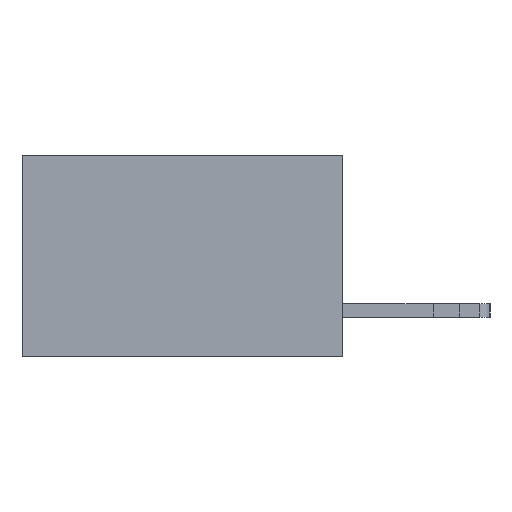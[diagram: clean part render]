
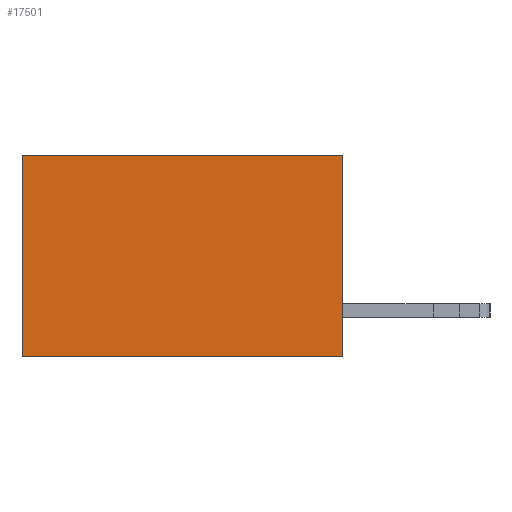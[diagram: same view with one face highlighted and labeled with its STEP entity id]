
A CAD part, left-side view. The second image highlights one B-rep face of the part: STEP entity #17501.
In plain terms, the highlighted planar face has unit normal (-1, 0, 0).
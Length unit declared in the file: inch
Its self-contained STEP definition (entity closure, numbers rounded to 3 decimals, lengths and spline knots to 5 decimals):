
#736 = VERTEX_POINT ( 'NONE', #9487 ) ;
#1729 = EDGE_CURVE ( 'NONE', #8625, #7861, #22455, .T. ) ;
#1842 = CARTESIAN_POINT ( 'NONE',  ( 0.277, 0., -0.37 ) ) ;
#3627 = CARTESIAN_POINT ( 'NONE',  ( 0.277, 0., -0.37 ) ) ;
#3672 = CARTESIAN_POINT ( 'NONE',  ( 0.277, 0.59, -0.37 ) ) ;
#3812 = DIRECTION ( 'NONE',  ( 0., 0., -1. ) ) ;
#3881 = CARTESIAN_POINT ( 'NONE',  ( 0.277, 0.59, 0. ) ) ;
#6607 = EDGE_CURVE ( 'NONE', #736, #9971, #23410, .T. ) ;
#7861 = VERTEX_POINT ( 'NONE', #3672 ) ;
#8625 = VERTEX_POINT ( 'NONE', #3881 ) ;
#8649 = VECTOR ( 'NONE', #17590, 39.37008 ) ;
#8766 = AXIS2_PLACEMENT_3D ( 'NONE', #1842, #15333, #3812 ) ;
#9177 = EDGE_CURVE ( 'NONE', #9971, #7861, #24227, .T. ) ;
#9293 = CARTESIAN_POINT ( 'NONE',  ( 0.277, 0., -0.37 ) ) ;
#9487 = CARTESIAN_POINT ( 'NONE',  ( 0.277, 0., 0. ) ) ;
#9596 = PLANE ( 'NONE',  #8766 ) ;
#9971 = VERTEX_POINT ( 'NONE', #3627 ) ;
#12658 = ORIENTED_EDGE ( 'NONE', *, *, #12904, .T. ) ;
#12904 = EDGE_CURVE ( 'NONE', #736, #8625, #14355, .T. ) ;
#13796 = CARTESIAN_POINT ( 'NONE',  ( 0.277, 0., 0. ) ) ;
#13883 = ORIENTED_EDGE ( 'NONE', *, *, #1729, .T. ) ;
#14211 = VECTOR ( 'NONE', #16876, 39.37008 ) ;
#14355 = LINE ( 'NONE', #13796, #8649 ) ;
#15333 = DIRECTION ( 'NONE',  ( 1., 0., 0. ) ) ;
#15438 = CARTESIAN_POINT ( 'NONE',  ( 0.277, 0.59, -0.37 ) ) ;
#15582 = DIRECTION ( 'NONE',  ( 0., 0., -1. ) ) ;
#15646 = VECTOR ( 'NONE', #16038, 39.37008 ) ;
#16038 = DIRECTION ( 'NONE',  ( 0., 0., -1. ) ) ;
#16876 = DIRECTION ( 'NONE',  ( 0., 1., 0. ) ) ;
#17501 = ADVANCED_FACE ( 'NONE', ( #18291 ), #9596, .F. ) ;
#17590 = DIRECTION ( 'NONE',  ( 0., 1., 0. ) ) ;
#18291 = FACE_OUTER_BOUND ( 'NONE', #22508, .T. ) ;
#18415 = VECTOR ( 'NONE', #15582, 39.37008 ) ;
#21907 = ORIENTED_EDGE ( 'NONE', *, *, #9177, .F. ) ;
#22455 = LINE ( 'NONE', #15438, #15646 ) ;
#22508 = EDGE_LOOP ( 'NONE', ( #13883, #21907, #23242, #12658 ) ) ;
#23109 = CARTESIAN_POINT ( 'NONE',  ( 0.277, 0., -0.37 ) ) ;
#23242 = ORIENTED_EDGE ( 'NONE', *, *, #6607, .F. ) ;
#23410 = LINE ( 'NONE', #23109, #18415 ) ;
#24227 = LINE ( 'NONE', #9293, #14211 ) ;
